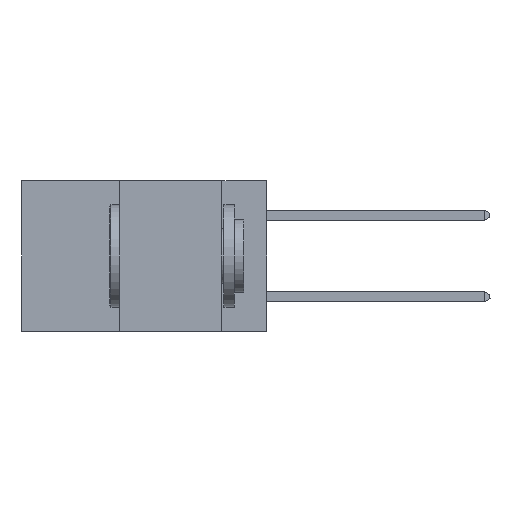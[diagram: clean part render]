
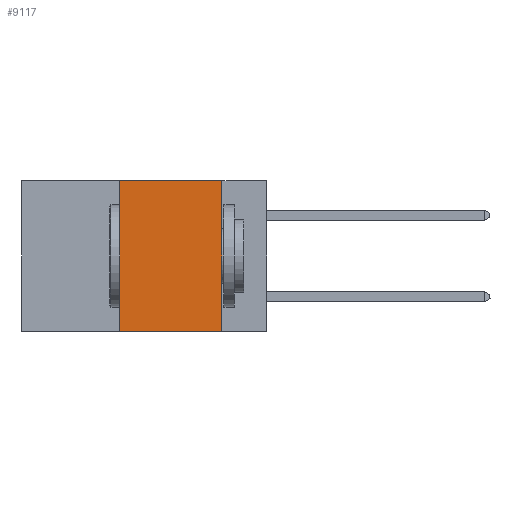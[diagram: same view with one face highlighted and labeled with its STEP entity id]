
A CAD part, left-side view. The second image highlights one B-rep face of the part: STEP entity #9117.
In plain terms, the highlighted planar face has unit normal (-1, 0, 0).
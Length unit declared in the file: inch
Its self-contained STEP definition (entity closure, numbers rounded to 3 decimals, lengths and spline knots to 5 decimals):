
#2045 = ORIENTED_EDGE ( 'NONE', *, *, #2673, .F. ) ;
#2673 = EDGE_CURVE ( 'NONE', #31128, #13421, #17773, .T. ) ;
#3884 = LINE ( 'NONE', #28676, #25316 ) ;
#4275 = CARTESIAN_POINT ( 'NONE',  ( 0., 0.11, -0.37 ) ) ;
#4747 = CARTESIAN_POINT ( 'NONE',  ( 0., 0.36, 0. ) ) ;
#9117 = ADVANCED_FACE ( 'NONE', ( #17495 ), #14447, .F. ) ;
#9500 = ORIENTED_EDGE ( 'NONE', *, *, #10642, .T. ) ;
#10642 = EDGE_CURVE ( 'NONE', #20999, #13421, #25175, .T. ) ;
#11055 = VECTOR ( 'NONE', #33280, 39.37008 ) ;
#11493 = CARTESIAN_POINT ( 'NONE',  ( 0., 0.6, 0. ) ) ;
#11911 = AXIS2_PLACEMENT_3D ( 'NONE', #11493, #33298, #39375 ) ;
#13114 = VECTOR ( 'NONE', #32263, 39.37008 ) ;
#13421 = VERTEX_POINT ( 'NONE', #4275 ) ;
#14086 = EDGE_CURVE ( 'NONE', #20999, #39277, #27746, .T. ) ;
#14447 = PLANE ( 'NONE',  #11911 ) ;
#17275 = CARTESIAN_POINT ( 'NONE',  ( 0., 0.36, 0. ) ) ;
#17495 = FACE_OUTER_BOUND ( 'NONE', #29715, .T. ) ;
#17773 = LINE ( 'NONE', #38957, #40207 ) ;
#19210 = ORIENTED_EDGE ( 'NONE', *, *, #14086, .F. ) ;
#20999 = VERTEX_POINT ( 'NONE', #24558 ) ;
#23782 = EDGE_CURVE ( 'NONE', #39277, #31128, #3884, .T. ) ;
#24558 = CARTESIAN_POINT ( 'NONE',  ( 0., 0.36, -0.37 ) ) ;
#25175 = LINE ( 'NONE', #36923, #11055 ) ;
#25316 = VECTOR ( 'NONE', #38174, 39.37008 ) ;
#27746 = LINE ( 'NONE', #4747, #13114 ) ;
#28360 = ORIENTED_EDGE ( 'NONE', *, *, #23782, .F. ) ;
#28676 = CARTESIAN_POINT ( 'NONE',  ( 0., 0.6, 0. ) ) ;
#29194 = DIRECTION ( 'NONE',  ( 0., 0., -1. ) ) ;
#29715 = EDGE_LOOP ( 'NONE', ( #2045, #28360, #19210, #9500 ) ) ;
#31128 = VERTEX_POINT ( 'NONE', #40107 ) ;
#32263 = DIRECTION ( 'NONE',  ( 0., 0., 1. ) ) ;
#33280 = DIRECTION ( 'NONE',  ( 0., -1., 0. ) ) ;
#33298 = DIRECTION ( 'NONE',  ( 1., 0., 0. ) ) ;
#36923 = CARTESIAN_POINT ( 'NONE',  ( 0., 0.6, -0.37 ) ) ;
#38174 = DIRECTION ( 'NONE',  ( 0., -1., 0. ) ) ;
#38957 = CARTESIAN_POINT ( 'NONE',  ( 0., 0.11, 0. ) ) ;
#39277 = VERTEX_POINT ( 'NONE', #17275 ) ;
#39375 = DIRECTION ( 'NONE',  ( 0., 0., -1. ) ) ;
#40107 = CARTESIAN_POINT ( 'NONE',  ( 0., 0.11, 0. ) ) ;
#40207 = VECTOR ( 'NONE', #29194, 39.37008 ) ;
